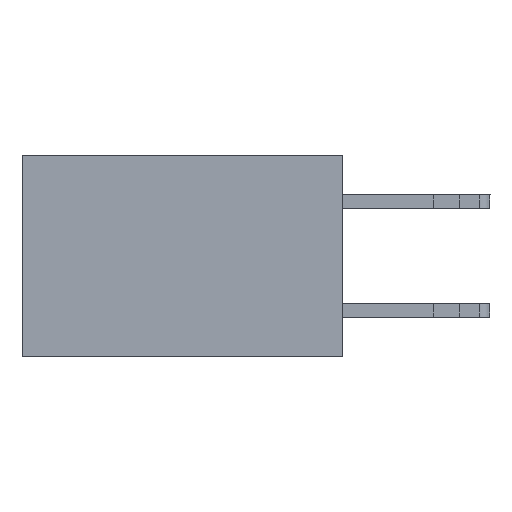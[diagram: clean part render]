
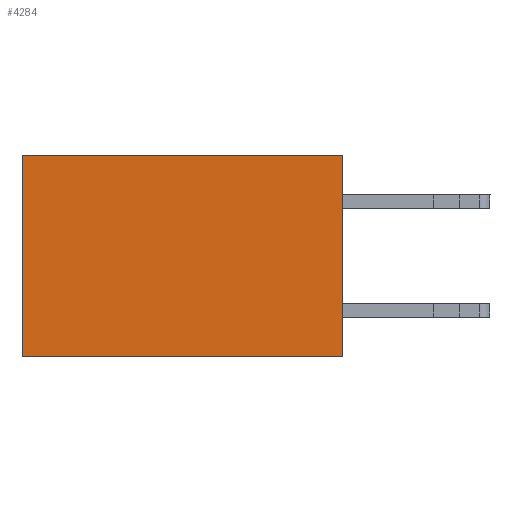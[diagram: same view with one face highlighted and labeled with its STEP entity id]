
A CAD part, left-side view. The second image highlights one B-rep face of the part: STEP entity #4284.
In plain terms, the highlighted planar face has unit normal (-1, 0, 0).
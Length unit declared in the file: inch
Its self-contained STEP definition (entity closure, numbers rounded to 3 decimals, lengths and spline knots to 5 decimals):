
#390 = VERTEX_POINT ( 'NONE', #1861 ) ;
#1861 = CARTESIAN_POINT ( 'NONE',  ( 0.277, 0., -0.37 ) ) ;
#1991 = CARTESIAN_POINT ( 'NONE',  ( 0.277, 0., -0.37 ) ) ;
#2678 = EDGE_CURVE ( 'NONE', #13005, #3928, #4110, .T. ) ;
#2787 = CARTESIAN_POINT ( 'NONE',  ( 0.277, 0., 0. ) ) ;
#2868 = VECTOR ( 'NONE', #9656, 39.37008 ) ;
#3779 = LINE ( 'NONE', #3967, #7543 ) ;
#3928 = VERTEX_POINT ( 'NONE', #10984 ) ;
#3967 = CARTESIAN_POINT ( 'NONE',  ( 0.277, 0.59, -0.37 ) ) ;
#4011 = CARTESIAN_POINT ( 'NONE',  ( 0.277, 0., -0.37 ) ) ;
#4110 = LINE ( 'NONE', #2787, #5237 ) ;
#4284 = ADVANCED_FACE ( 'NONE', ( #4958 ), #14712, .F. ) ;
#4958 = FACE_OUTER_BOUND ( 'NONE', #12935, .T. ) ;
#5237 = VECTOR ( 'NONE', #9652, 39.37008 ) ;
#5368 = ORIENTED_EDGE ( 'NONE', *, *, #12043, .F. ) ;
#6914 = LINE ( 'NONE', #4011, #2868 ) ;
#6926 = DIRECTION ( 'NONE',  ( 0., 1., 0. ) ) ;
#7543 = VECTOR ( 'NONE', #13918, 39.37008 ) ;
#7676 = DIRECTION ( 'NONE',  ( 1., 0., 0. ) ) ;
#8341 = ORIENTED_EDGE ( 'NONE', *, *, #17347, .F. ) ;
#8491 = CARTESIAN_POINT ( 'NONE',  ( 0.277, 0., -0.37 ) ) ;
#9652 = DIRECTION ( 'NONE',  ( 0., 1., 0. ) ) ;
#9656 = DIRECTION ( 'NONE',  ( 0., 0., -1. ) ) ;
#10021 = ORIENTED_EDGE ( 'NONE', *, *, #2678, .T. ) ;
#10064 = CARTESIAN_POINT ( 'NONE',  ( 0.277, 0.59, -0.37 ) ) ;
#10100 = EDGE_CURVE ( 'NONE', #3928, #10745, #3779, .T. ) ;
#10745 = VERTEX_POINT ( 'NONE', #10064 ) ;
#10984 = CARTESIAN_POINT ( 'NONE',  ( 0.277, 0.59, 0. ) ) ;
#12043 = EDGE_CURVE ( 'NONE', #390, #10745, #14436, .T. ) ;
#12935 = EDGE_LOOP ( 'NONE', ( #17718, #5368, #8341, #10021 ) ) ;
#13005 = VERTEX_POINT ( 'NONE', #14388 ) ;
#13334 = DIRECTION ( 'NONE',  ( 0., 0., -1. ) ) ;
#13918 = DIRECTION ( 'NONE',  ( 0., 0., -1. ) ) ;
#14388 = CARTESIAN_POINT ( 'NONE',  ( 0.277, 0., 0. ) ) ;
#14436 = LINE ( 'NONE', #8491, #15675 ) ;
#14712 = PLANE ( 'NONE',  #14929 ) ;
#14929 = AXIS2_PLACEMENT_3D ( 'NONE', #1991, #7676, #13334 ) ;
#15675 = VECTOR ( 'NONE', #6926, 39.37008 ) ;
#17347 = EDGE_CURVE ( 'NONE', #13005, #390, #6914, .T. ) ;
#17718 = ORIENTED_EDGE ( 'NONE', *, *, #10100, .T. ) ;
